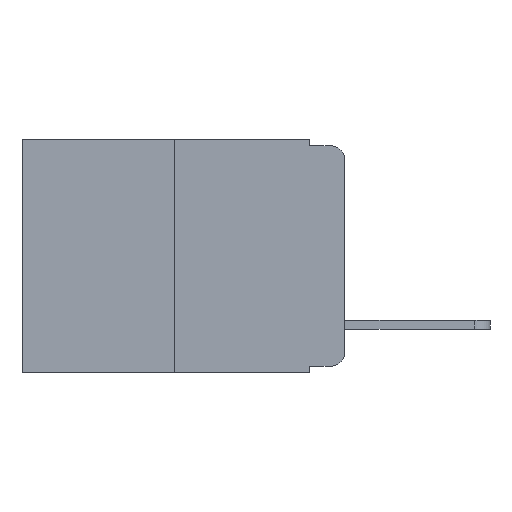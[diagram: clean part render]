
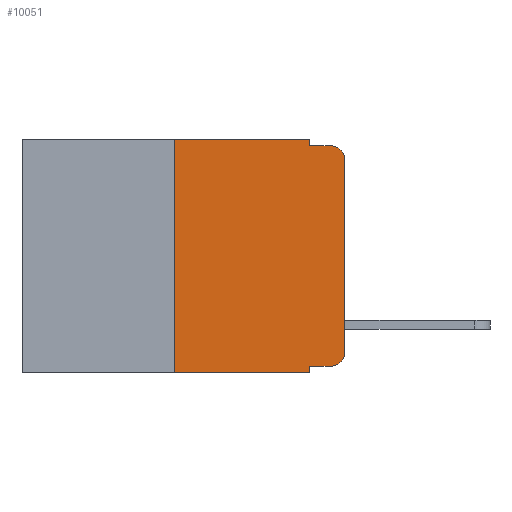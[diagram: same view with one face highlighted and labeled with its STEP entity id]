
A CAD part, left-side view. The second image highlights one B-rep face of the part: STEP entity #10051.
In plain terms, the highlighted planar face has unit normal (-1, 0, 0).
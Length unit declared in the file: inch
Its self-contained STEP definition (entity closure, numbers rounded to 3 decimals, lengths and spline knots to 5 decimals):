
#868 = VERTEX_POINT ( 'NONE', #10231 ) ;
#1021 = CARTESIAN_POINT ( 'NONE',  ( 0., 0.051, 0. ) ) ;
#1124 = DIRECTION ( 'NONE',  ( 0., 0., -1. ) ) ;
#1172 = DIRECTION ( 'NONE',  ( -1., 0., 0. ) ) ;
#1178 = CARTESIAN_POINT ( 'NONE',  ( 0., 0.02, -0.03 ) ) ;
#1199 = EDGE_CURVE ( 'NONE', #7197, #868, #11576, .T. ) ;
#1329 = EDGE_LOOP ( 'NONE', ( #8676, #8716, #8697, #8727, #8742, #8731, #8744, #8769, #8790, #9072 ) ) ;
#1772 = EDGE_CURVE ( 'NONE', #7197, #7982, #10105, .T. ) ;
#1775 = EDGE_CURVE ( 'NONE', #5976, #6941, #2887, .T. ) ;
#1789 = EDGE_CURVE ( 'NONE', #11682, #1924, #7368, .T. ) ;
#1791 = EDGE_CURVE ( 'NONE', #11682, #868, #2552, .T. ) ;
#1808 = EDGE_CURVE ( 'NONE', #1924, #6732, #11844, .T. ) ;
#1924 = VERTEX_POINT ( 'NONE', #6758 ) ;
#1944 = VERTEX_POINT ( 'NONE', #9584 ) ;
#1962 = CIRCLE ( 'NONE', #7358, 0.02 ) ;
#2039 = CARTESIAN_POINT ( 'NONE',  ( 0., 0.25, -0.343 ) ) ;
#2123 = CARTESIAN_POINT ( 'NONE',  ( 0., 0.473, -0.343 ) ) ;
#2249 = DIRECTION ( 'NONE',  ( 0., -1., 0. ) ) ;
#2341 = DIRECTION ( 'NONE',  ( -1., 0., 0. ) ) ;
#2382 = CARTESIAN_POINT ( 'NONE',  ( 0., 0.051, -0.01 ) ) ;
#2552 = LINE ( 'NONE', #11868, #7943 ) ;
#2573 = VECTOR ( 'NONE', #4687, 39.37008 ) ;
#2887 = LINE ( 'NONE', #1021, #12084 ) ;
#2974 = DIRECTION ( 'NONE',  ( 0., 0., -1. ) ) ;
#3516 = DIRECTION ( 'NONE',  ( 0., 0., -1. ) ) ;
#4051 = CARTESIAN_POINT ( 'NONE',  ( 0., 0.051, -0.333 ) ) ;
#4320 = DIRECTION ( 'NONE',  ( 0., -1., 0. ) ) ;
#4600 = AXIS2_PLACEMENT_3D ( 'NONE', #6747, #2341, #2974 ) ;
#4651 = CARTESIAN_POINT ( 'NONE',  ( 0., 0.473, 0. ) ) ;
#4687 = DIRECTION ( 'NONE',  ( 0., 0., 1. ) ) ;
#4725 = CARTESIAN_POINT ( 'NONE',  ( 0., 0., 0. ) ) ;
#4923 = VECTOR ( 'NONE', #12239, 39.37008 ) ;
#5227 = VECTOR ( 'NONE', #10433, 39.37008 ) ;
#5976 = VERTEX_POINT ( 'NONE', #9872 ) ;
#6542 = VERTEX_POINT ( 'NONE', #11190 ) ;
#6612 = CARTESIAN_POINT ( 'NONE',  ( 0., 0., -0.313 ) ) ;
#6635 = EDGE_CURVE ( 'NONE', #6941, #6542, #10616, .T. ) ;
#6732 = VERTEX_POINT ( 'NONE', #6612 ) ;
#6747 = CARTESIAN_POINT ( 'NONE',  ( 0., 0.02, -0.313 ) ) ;
#6758 = CARTESIAN_POINT ( 'NONE',  ( 0., 0.02, -0.333 ) ) ;
#6833 = VECTOR ( 'NONE', #8821, 39.37008 ) ;
#6941 = VERTEX_POINT ( 'NONE', #12172 ) ;
#7197 = VERTEX_POINT ( 'NONE', #2039 ) ;
#7358 = AXIS2_PLACEMENT_3D ( 'NONE', #1178, #1172, #1124 ) ;
#7368 = LINE ( 'NONE', #11908, #4923 ) ;
#7669 = LINE ( 'NONE', #4725, #2573 ) ;
#7943 = VECTOR ( 'NONE', #3516, 39.37008 ) ;
#7982 = VERTEX_POINT ( 'NONE', #11711 ) ;
#8099 = EDGE_CURVE ( 'NONE', #1944, #6542, #1962, .T. ) ;
#8463 = VECTOR ( 'NONE', #2249, 39.37008 ) ;
#8676 = ORIENTED_EDGE ( 'NONE', *, *, #10886, .T. ) ;
#8697 = ORIENTED_EDGE ( 'NONE', *, *, #6635, .F. ) ;
#8716 = ORIENTED_EDGE ( 'NONE', *, *, #8099, .T. ) ;
#8727 = ORIENTED_EDGE ( 'NONE', *, *, #1775, .F. ) ;
#8731 = ORIENTED_EDGE ( 'NONE', *, *, #1772, .F. ) ;
#8742 = ORIENTED_EDGE ( 'NONE', *, *, #11661, .F. ) ;
#8744 = ORIENTED_EDGE ( 'NONE', *, *, #1199, .T. ) ;
#8769 = ORIENTED_EDGE ( 'NONE', *, *, #1791, .F. ) ;
#8790 = ORIENTED_EDGE ( 'NONE', *, *, #1789, .T. ) ;
#8821 = DIRECTION ( 'NONE',  ( 0., -1., 0. ) ) ;
#9051 = FACE_OUTER_BOUND ( 'NONE', #1329, .T. ) ;
#9072 = ORIENTED_EDGE ( 'NONE', *, *, #1808, .T. ) ;
#9584 = CARTESIAN_POINT ( 'NONE',  ( 0., 0., -0.03 ) ) ;
#9644 = AXIS2_PLACEMENT_3D ( 'NONE', #10483, #10424, #10408 ) ;
#9872 = CARTESIAN_POINT ( 'NONE',  ( 0., 0.051, 0. ) ) ;
#10051 = ADVANCED_FACE ( 'NONE', ( #9051 ), #10550, .F. ) ;
#10105 = LINE ( 'NONE', #10346, #5227 ) ;
#10231 = CARTESIAN_POINT ( 'NONE',  ( 0., 0.051, -0.343 ) ) ;
#10346 = CARTESIAN_POINT ( 'NONE',  ( 0., 0.25, 0. ) ) ;
#10401 = VECTOR ( 'NONE', #4320, 39.37008 ) ;
#10408 = DIRECTION ( 'NONE',  ( 0., 0., -1. ) ) ;
#10424 = DIRECTION ( 'NONE',  ( 1., 0., 0. ) ) ;
#10433 = DIRECTION ( 'NONE',  ( 0., 0., 1. ) ) ;
#10483 = CARTESIAN_POINT ( 'NONE',  ( 0., 0.473, 0. ) ) ;
#10550 = PLANE ( 'NONE',  #9644 ) ;
#10616 = LINE ( 'NONE', #2382, #8463 ) ;
#10684 = DIRECTION ( 'NONE',  ( 0., 0., -1. ) ) ;
#10886 = EDGE_CURVE ( 'NONE', #6732, #1944, #7669, .T. ) ;
#11190 = CARTESIAN_POINT ( 'NONE',  ( 0., 0.02, -0.01 ) ) ;
#11576 = LINE ( 'NONE', #2123, #6833 ) ;
#11661 = EDGE_CURVE ( 'NONE', #7982, #5976, #12385, .T. ) ;
#11682 = VERTEX_POINT ( 'NONE', #4051 ) ;
#11711 = CARTESIAN_POINT ( 'NONE',  ( 0., 0.25, 0. ) ) ;
#11844 = CIRCLE ( 'NONE', #4600, 0.02 ) ;
#11868 = CARTESIAN_POINT ( 'NONE',  ( 0., 0.051, 0. ) ) ;
#11908 = CARTESIAN_POINT ( 'NONE',  ( 0., 0.051, -0.333 ) ) ;
#12084 = VECTOR ( 'NONE', #10684, 39.37008 ) ;
#12172 = CARTESIAN_POINT ( 'NONE',  ( 0., 0.051, -0.01 ) ) ;
#12239 = DIRECTION ( 'NONE',  ( 0., -1., 0. ) ) ;
#12385 = LINE ( 'NONE', #4651, #10401 ) ;
